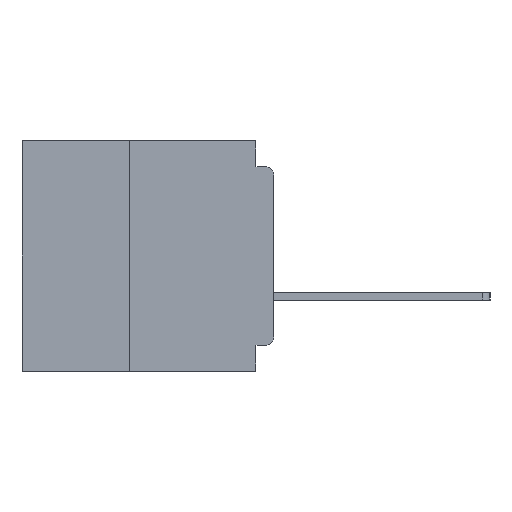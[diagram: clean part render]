
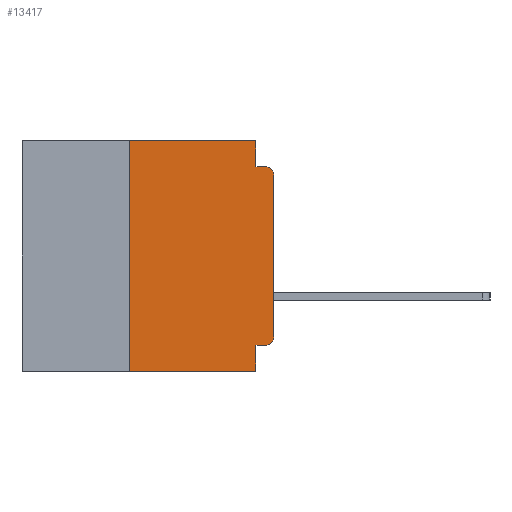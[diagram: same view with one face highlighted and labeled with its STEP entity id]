
A CAD part, left-side view. The second image highlights one B-rep face of the part: STEP entity #13417.
In plain terms, the highlighted planar face has unit normal (-1, 0, 0).
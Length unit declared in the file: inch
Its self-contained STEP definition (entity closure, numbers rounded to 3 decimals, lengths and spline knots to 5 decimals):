
#680 = PLANE ( 'NONE',  #1681 ) ;
#1681 = AXIS2_PLACEMENT_3D ( 'NONE', #35678, #3890, #26283 ) ;
#3260 = LINE ( 'NONE', #32187, #37174 ) ;
#3712 = CIRCLE ( 'NONE', #24785, 0.015 ) ;
#3841 = CARTESIAN_POINT ( 'NONE',  ( 0., 0.015, -0.06 ) ) ;
#3890 = DIRECTION ( 'NONE',  ( 1., 0., 0. ) ) ;
#4588 = EDGE_CURVE ( 'NONE', #35244, #13283, #12965, .T. ) ;
#4844 = DIRECTION ( 'NONE',  ( 0., -1., 0. ) ) ;
#4951 = VERTEX_POINT ( 'NONE', #13313 ) ;
#5162 = VERTEX_POINT ( 'NONE', #33308 ) ;
#5694 = ORIENTED_EDGE ( 'NONE', *, *, #6401, .F. ) ;
#5724 = EDGE_LOOP ( 'NONE', ( #19935, #11041, #11972, #7770, #5694, #29221, #38433, #12555, #26863, #13046 ) ) ;
#6401 = EDGE_CURVE ( 'NONE', #32761, #21640, #27352, .T. ) ;
#6962 = LINE ( 'NONE', #23237, #14544 ) ;
#7052 = DIRECTION ( 'NONE',  ( 0., 0., -1. ) ) ;
#7770 = ORIENTED_EDGE ( 'NONE', *, *, #37678, .F. ) ;
#8623 = LINE ( 'NONE', #9267, #24647 ) ;
#9267 = CARTESIAN_POINT ( 'NONE',  ( 0., 0.25, -0.4 ) ) ;
#10228 = EDGE_CURVE ( 'NONE', #13283, #25860, #27022, .T. ) ;
#10484 = DIRECTION ( 'NONE',  ( 0., -1., 0. ) ) ;
#11041 = ORIENTED_EDGE ( 'NONE', *, *, #15372, .T. ) ;
#11642 = DIRECTION ( 'NONE',  ( -1., 0., 0. ) ) ;
#11972 = ORIENTED_EDGE ( 'NONE', *, *, #38735, .F. ) ;
#12555 = ORIENTED_EDGE ( 'NONE', *, *, #27078, .F. ) ;
#12965 = CIRCLE ( 'NONE', #19428, 0.015 ) ;
#13046 = ORIENTED_EDGE ( 'NONE', *, *, #4588, .T. ) ;
#13283 = VERTEX_POINT ( 'NONE', #19069 ) ;
#13313 = CARTESIAN_POINT ( 'NONE',  ( 0., 0.031, -0.045 ) ) ;
#13396 = CARTESIAN_POINT ( 'NONE',  ( 0., 0.031, -0.4 ) ) ;
#13417 = ADVANCED_FACE ( 'NONE', ( #36311 ), #680, .F. ) ;
#14544 = VECTOR ( 'NONE', #10484, 39.37008 ) ;
#15159 = VECTOR ( 'NONE', #35613, 39.37008 ) ;
#15372 = EDGE_CURVE ( 'NONE', #25860, #31886, #3712, .T. ) ;
#16348 = DIRECTION ( 'NONE',  ( 0., 0., -1. ) ) ;
#17555 = VECTOR ( 'NONE', #31839, 39.37008 ) ;
#17747 = CARTESIAN_POINT ( 'NONE',  ( 0., 0.437, 0. ) ) ;
#18893 = VECTOR ( 'NONE', #4844, 39.37008 ) ;
#19069 = CARTESIAN_POINT ( 'NONE',  ( 0., 0., -0.34 ) ) ;
#19238 = CARTESIAN_POINT ( 'NONE',  ( 0., 0., 0. ) ) ;
#19428 = AXIS2_PLACEMENT_3D ( 'NONE', #30711, #11642, #33909 ) ;
#19928 = VECTOR ( 'NONE', #24426, 39.37008 ) ;
#19935 = ORIENTED_EDGE ( 'NONE', *, *, #10228, .T. ) ;
#20256 = VERTEX_POINT ( 'NONE', #23036 ) ;
#21640 = VERTEX_POINT ( 'NONE', #33145 ) ;
#21778 = EDGE_CURVE ( 'NONE', #35244, #29721, #28365, .T. ) ;
#23036 = CARTESIAN_POINT ( 'NONE',  ( 0., 0.031, -0.4 ) ) ;
#23237 = CARTESIAN_POINT ( 'NONE',  ( 0., 0.437, -0.4 ) ) ;
#24426 = DIRECTION ( 'NONE',  ( 0., 1., 0. ) ) ;
#24647 = VECTOR ( 'NONE', #34762, 39.37008 ) ;
#24785 = AXIS2_PLACEMENT_3D ( 'NONE', #3841, #26238, #7052 ) ;
#25860 = VERTEX_POINT ( 'NONE', #41079 ) ;
#26238 = DIRECTION ( 'NONE',  ( -1., 0., 0. ) ) ;
#26283 = DIRECTION ( 'NONE',  ( 0., 0., -1. ) ) ;
#26863 = ORIENTED_EDGE ( 'NONE', *, *, #21778, .F. ) ;
#27022 = LINE ( 'NONE', #19238, #17555 ) ;
#27078 = EDGE_CURVE ( 'NONE', #29721, #20256, #38465, .T. ) ;
#27352 = LINE ( 'NONE', #17747, #18893 ) ;
#28365 = LINE ( 'NONE', #33834, #19928 ) ;
#28736 = VECTOR ( 'NONE', #34868, 39.37008 ) ;
#29181 = EDGE_CURVE ( 'NONE', #5162, #20256, #6962, .T. ) ;
#29221 = ORIENTED_EDGE ( 'NONE', *, *, #31300, .F. ) ;
#29713 = LINE ( 'NONE', #37920, #28736 ) ;
#29721 = VERTEX_POINT ( 'NONE', #36206 ) ;
#30711 = CARTESIAN_POINT ( 'NONE',  ( 0., 0.015, -0.34 ) ) ;
#31103 = CARTESIAN_POINT ( 'NONE',  ( 0., 0.015, -0.045 ) ) ;
#31300 = EDGE_CURVE ( 'NONE', #5162, #32761, #8623, .T. ) ;
#31839 = DIRECTION ( 'NONE',  ( 0., 0., 1. ) ) ;
#31886 = VERTEX_POINT ( 'NONE', #31103 ) ;
#32187 = CARTESIAN_POINT ( 'NONE',  ( 0., 0.031, 0. ) ) ;
#32761 = VERTEX_POINT ( 'NONE', #39042 ) ;
#32822 = CARTESIAN_POINT ( 'NONE',  ( 0., 0.015, -0.355 ) ) ;
#33145 = CARTESIAN_POINT ( 'NONE',  ( 0., 0.031, 0. ) ) ;
#33308 = CARTESIAN_POINT ( 'NONE',  ( 0., 0.25, -0.4 ) ) ;
#33834 = CARTESIAN_POINT ( 'NONE',  ( 0., 0., -0.355 ) ) ;
#33909 = DIRECTION ( 'NONE',  ( 0., 0., -1. ) ) ;
#34762 = DIRECTION ( 'NONE',  ( 0., 0., 1. ) ) ;
#34868 = DIRECTION ( 'NONE',  ( 0., -1., 0. ) ) ;
#35244 = VERTEX_POINT ( 'NONE', #32822 ) ;
#35613 = DIRECTION ( 'NONE',  ( 0., 0., -1. ) ) ;
#35678 = CARTESIAN_POINT ( 'NONE',  ( 0., 0.437, 0. ) ) ;
#36206 = CARTESIAN_POINT ( 'NONE',  ( 0., 0.031, -0.355 ) ) ;
#36311 = FACE_OUTER_BOUND ( 'NONE', #5724, .T. ) ;
#37174 = VECTOR ( 'NONE', #16348, 39.37008 ) ;
#37678 = EDGE_CURVE ( 'NONE', #21640, #4951, #3260, .T. ) ;
#37920 = CARTESIAN_POINT ( 'NONE',  ( 0., 0., -0.045 ) ) ;
#38433 = ORIENTED_EDGE ( 'NONE', *, *, #29181, .T. ) ;
#38465 = LINE ( 'NONE', #13396, #15159 ) ;
#38735 = EDGE_CURVE ( 'NONE', #4951, #31886, #29713, .T. ) ;
#39042 = CARTESIAN_POINT ( 'NONE',  ( 0., 0.25, 0. ) ) ;
#41079 = CARTESIAN_POINT ( 'NONE',  ( 0., 0., -0.06 ) ) ;
